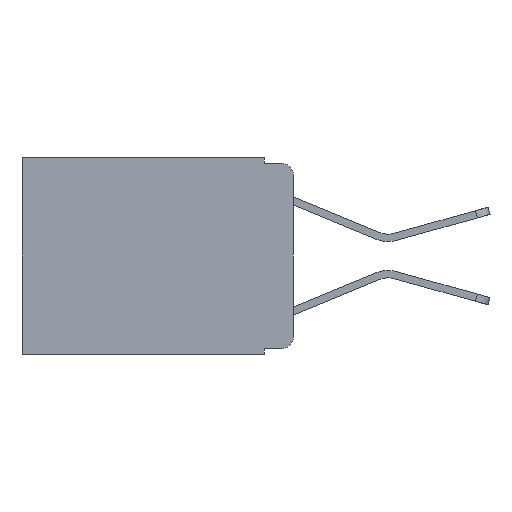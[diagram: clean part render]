
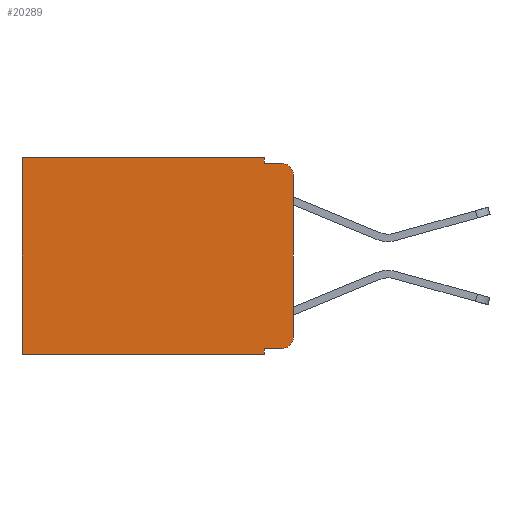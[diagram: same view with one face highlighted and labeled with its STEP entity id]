
A CAD part, left-side view. The second image highlights one B-rep face of the part: STEP entity #20289.
In plain terms, the highlighted planar face has unit normal (-1, 0, 0).
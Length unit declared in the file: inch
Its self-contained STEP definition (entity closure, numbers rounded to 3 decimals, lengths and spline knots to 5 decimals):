
#568 = VERTEX_POINT ( 'NONE', #9834 ) ;
#784 = LINE ( 'NONE', #18323, #13047 ) ;
#1042 = CARTESIAN_POINT ( 'NONE',  ( 0.298, 0., -0.03 ) ) ;
#1084 = VECTOR ( 'NONE', #1816, 39.37008 ) ;
#1096 = ORIENTED_EDGE ( 'NONE', *, *, #9197, .F. ) ;
#1520 = CARTESIAN_POINT ( 'NONE',  ( 0.298, 0., -0.313 ) ) ;
#1631 = ORIENTED_EDGE ( 'NONE', *, *, #19078, .T. ) ;
#1816 = DIRECTION ( 'NONE',  ( 0., -1., 0. ) ) ;
#1904 = CARTESIAN_POINT ( 'NONE',  ( 0.298, 0.051, -0.333 ) ) ;
#2073 = LINE ( 'NONE', #10811, #18478 ) ;
#2117 = VERTEX_POINT ( 'NONE', #3709 ) ;
#2651 = AXIS2_PLACEMENT_3D ( 'NONE', #7008, #18070, #8637 ) ;
#2923 = VERTEX_POINT ( 'NONE', #6080 ) ;
#2991 = LINE ( 'NONE', #14916, #10985 ) ;
#3211 = EDGE_CURVE ( 'NONE', #568, #12276, #6887, .T. ) ;
#3236 = EDGE_CURVE ( 'NONE', #4616, #15506, #5376, .T. ) ;
#3610 = ORIENTED_EDGE ( 'NONE', *, *, #3211, .T. ) ;
#3709 = CARTESIAN_POINT ( 'NONE',  ( 0.298, 0.02, -0.01 ) ) ;
#3771 = DIRECTION ( 'NONE',  ( 0., 0., -1. ) ) ;
#4277 = CARTESIAN_POINT ( 'NONE',  ( 0.298, 0., -0.343 ) ) ;
#4431 = CARTESIAN_POINT ( 'NONE',  ( 0.298, 0., 0. ) ) ;
#4616 = VERTEX_POINT ( 'NONE', #9899 ) ;
#4631 = ORIENTED_EDGE ( 'NONE', *, *, #15420, .F. ) ;
#4822 = FACE_OUTER_BOUND ( 'NONE', #9058, .T. ) ;
#5126 = VERTEX_POINT ( 'NONE', #1520 ) ;
#5216 = CARTESIAN_POINT ( 'NONE',  ( 0.298, 0., 0. ) ) ;
#5376 = LINE ( 'NONE', #4431, #17545 ) ;
#5642 = DIRECTION ( 'NONE',  ( -1., 0., 0. ) ) ;
#5881 = DIRECTION ( 'NONE',  ( 0., 1., 0. ) ) ;
#5945 = EDGE_CURVE ( 'NONE', #14113, #5126, #13497, .T. ) ;
#6080 = CARTESIAN_POINT ( 'NONE',  ( 0.298, 0.473, -0.343 ) ) ;
#6172 = ORIENTED_EDGE ( 'NONE', *, *, #18932, .F. ) ;
#6848 = DIRECTION ( 'NONE',  ( 0., 0., -1. ) ) ;
#6877 = ORIENTED_EDGE ( 'NONE', *, *, #19773, .T. ) ;
#6887 = LINE ( 'NONE', #1904, #1084 ) ;
#7008 = CARTESIAN_POINT ( 'NONE',  ( 0.298, 0.02, -0.03 ) ) ;
#7036 = CARTESIAN_POINT ( 'NONE',  ( 0.298, 0., 0. ) ) ;
#7390 = ORIENTED_EDGE ( 'NONE', *, *, #5945, .F. ) ;
#8064 = EDGE_CURVE ( 'NONE', #12276, #5126, #19535, .T. ) ;
#8352 = AXIS2_PLACEMENT_3D ( 'NONE', #15181, #5642, #16760 ) ;
#8425 = ORIENTED_EDGE ( 'NONE', *, *, #11259, .F. ) ;
#8637 = DIRECTION ( 'NONE',  ( 0., 0., -1. ) ) ;
#8933 = ORIENTED_EDGE ( 'NONE', *, *, #8064, .T. ) ;
#9058 = EDGE_LOOP ( 'NONE', ( #7390, #6877, #4631, #1096, #17551, #1631, #8425, #6172, #3610, #8933 ) ) ;
#9197 = EDGE_CURVE ( 'NONE', #4616, #13274, #2991, .T. ) ;
#9324 = VECTOR ( 'NONE', #10192, 39.37008 ) ;
#9834 = CARTESIAN_POINT ( 'NONE',  ( 0.298, 0.051, -0.333 ) ) ;
#9899 = CARTESIAN_POINT ( 'NONE',  ( 0.298, 0.051, 0. ) ) ;
#10019 = VECTOR ( 'NONE', #12299, 39.37008 ) ;
#10192 = DIRECTION ( 'NONE',  ( 0., 0., -1. ) ) ;
#10811 = CARTESIAN_POINT ( 'NONE',  ( 0.298, 0.473, 0. ) ) ;
#10985 = VECTOR ( 'NONE', #3771, 39.37008 ) ;
#11259 = EDGE_CURVE ( 'NONE', #16293, #2923, #16594, .T. ) ;
#11465 = AXIS2_PLACEMENT_3D ( 'NONE', #5216, #16359, #6848 ) ;
#11789 = CARTESIAN_POINT ( 'NONE',  ( 0.298, 0.051, -0.01 ) ) ;
#11790 = CIRCLE ( 'NONE', #2651, 0.02 ) ;
#12276 = VERTEX_POINT ( 'NONE', #14801 ) ;
#12299 = DIRECTION ( 'NONE',  ( 0., -1., 0. ) ) ;
#12372 = VECTOR ( 'NONE', #5881, 39.37008 ) ;
#12491 = CARTESIAN_POINT ( 'NONE',  ( 0.298, 0.473, 0. ) ) ;
#13047 = VECTOR ( 'NONE', #18254, 39.37008 ) ;
#13147 = PLANE ( 'NONE',  #11465 ) ;
#13274 = VERTEX_POINT ( 'NONE', #11789 ) ;
#13497 = LINE ( 'NONE', #7036, #9324 ) ;
#13996 = DIRECTION ( 'NONE',  ( 0., 0., -1. ) ) ;
#14113 = VERTEX_POINT ( 'NONE', #1042 ) ;
#14801 = CARTESIAN_POINT ( 'NONE',  ( 0.298, 0.02, -0.333 ) ) ;
#14916 = CARTESIAN_POINT ( 'NONE',  ( 0.298, 0.051, 0. ) ) ;
#15181 = CARTESIAN_POINT ( 'NONE',  ( 0.298, 0.02, -0.313 ) ) ;
#15420 = EDGE_CURVE ( 'NONE', #13274, #2117, #18867, .T. ) ;
#15506 = VERTEX_POINT ( 'NONE', #12491 ) ;
#16293 = VERTEX_POINT ( 'NONE', #19061 ) ;
#16359 = DIRECTION ( 'NONE',  ( 1., 0., 0. ) ) ;
#16594 = LINE ( 'NONE', #4277, #12372 ) ;
#16760 = DIRECTION ( 'NONE',  ( 0., 0., -1. ) ) ;
#17545 = VECTOR ( 'NONE', #17809, 39.37008 ) ;
#17551 = ORIENTED_EDGE ( 'NONE', *, *, #3236, .T. ) ;
#17809 = DIRECTION ( 'NONE',  ( 0., 1., 0. ) ) ;
#18070 = DIRECTION ( 'NONE',  ( -1., 0., 0. ) ) ;
#18254 = DIRECTION ( 'NONE',  ( 0., 0., -1. ) ) ;
#18323 = CARTESIAN_POINT ( 'NONE',  ( 0.298, 0.051, 0. ) ) ;
#18478 = VECTOR ( 'NONE', #13996, 39.37008 ) ;
#18567 = CARTESIAN_POINT ( 'NONE',  ( 0.298, 0.051, -0.01 ) ) ;
#18867 = LINE ( 'NONE', #18567, #10019 ) ;
#18932 = EDGE_CURVE ( 'NONE', #568, #16293, #784, .T. ) ;
#19061 = CARTESIAN_POINT ( 'NONE',  ( 0.298, 0.051, -0.343 ) ) ;
#19078 = EDGE_CURVE ( 'NONE', #15506, #2923, #2073, .T. ) ;
#19535 = CIRCLE ( 'NONE', #8352, 0.02 ) ;
#19773 = EDGE_CURVE ( 'NONE', #14113, #2117, #11790, .T. ) ;
#20289 = ADVANCED_FACE ( 'NONE', ( #4822 ), #13147, .F. ) ;
